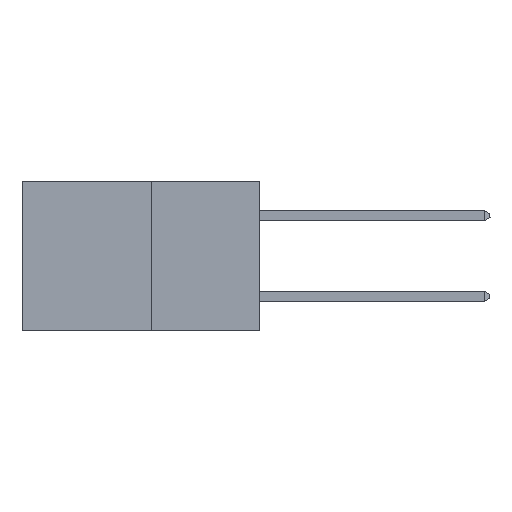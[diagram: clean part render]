
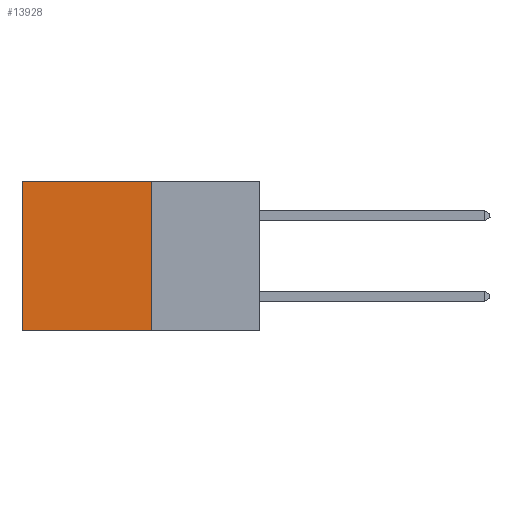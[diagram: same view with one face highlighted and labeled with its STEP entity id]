
A CAD part, left-side view. The second image highlights one B-rep face of the part: STEP entity #13928.
In plain terms, the highlighted planar face has unit normal (-1, 0, 0).
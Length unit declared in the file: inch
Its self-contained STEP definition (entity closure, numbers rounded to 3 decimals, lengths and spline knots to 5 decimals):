
#190 = EDGE_CURVE ( 'NONE', #4713, #26389, #25312, .T. ) ;
#2815 = VECTOR ( 'NONE', #17369, 39.37008 ) ;
#3020 = DIRECTION ( 'NONE',  ( 0., 0., -1. ) ) ;
#3487 = LINE ( 'NONE', #23505, #2815 ) ;
#4713 = VERTEX_POINT ( 'NONE', #15309 ) ;
#4972 = LINE ( 'NONE', #18026, #16426 ) ;
#5358 = CARTESIAN_POINT ( 'NONE',  ( 0.277, 0.27, 0. ) ) ;
#5372 = AXIS2_PLACEMENT_3D ( 'NONE', #22694, #10097, #24792 ) ;
#5730 = PLANE ( 'NONE',  #5372 ) ;
#5751 = LINE ( 'NONE', #5358, #17170 ) ;
#6756 = EDGE_CURVE ( 'NONE', #11425, #4713, #3487, .T. ) ;
#9179 = FACE_OUTER_BOUND ( 'NONE', #25872, .T. ) ;
#9618 = CARTESIAN_POINT ( 'NONE',  ( 0.277, 0.59, -0.37 ) ) ;
#9659 = DIRECTION ( 'NONE',  ( 0., 1., 0. ) ) ;
#10097 = DIRECTION ( 'NONE',  ( 1., 0., 0. ) ) ;
#11425 = VERTEX_POINT ( 'NONE', #22113 ) ;
#12475 = CARTESIAN_POINT ( 'NONE',  ( 0.277, 0.59, 0. ) ) ;
#13928 = ADVANCED_FACE ( 'NONE', ( #9179 ), #5730, .F. ) ;
#15016 = EDGE_CURVE ( 'NONE', #21531, #26389, #4972, .T. ) ;
#15309 = CARTESIAN_POINT ( 'NONE',  ( 0.277, 0.27, -0.37 ) ) ;
#15899 = DIRECTION ( 'NONE',  ( 0., 1., 0. ) ) ;
#16426 = VECTOR ( 'NONE', #3020, 39.37008 ) ;
#17170 = VECTOR ( 'NONE', #9659, 39.37008 ) ;
#17369 = DIRECTION ( 'NONE',  ( 0., 0., -1. ) ) ;
#17958 = ORIENTED_EDGE ( 'NONE', *, *, #190, .F. ) ;
#18026 = CARTESIAN_POINT ( 'NONE',  ( 0.277, 0.59, -0.37 ) ) ;
#18248 = ORIENTED_EDGE ( 'NONE', *, *, #6756, .F. ) ;
#19142 = VECTOR ( 'NONE', #15899, 39.37008 ) ;
#19360 = EDGE_CURVE ( 'NONE', #11425, #21531, #5751, .T. ) ;
#21357 = CARTESIAN_POINT ( 'NONE',  ( 0.277, 0.27, -0.37 ) ) ;
#21531 = VERTEX_POINT ( 'NONE', #12475 ) ;
#22113 = CARTESIAN_POINT ( 'NONE',  ( 0.277, 0.27, 0. ) ) ;
#22694 = CARTESIAN_POINT ( 'NONE',  ( 0.277, 0.27, -0.37 ) ) ;
#23505 = CARTESIAN_POINT ( 'NONE',  ( 0.277, 0.27, -0.37 ) ) ;
#23735 = ORIENTED_EDGE ( 'NONE', *, *, #19360, .T. ) ;
#24792 = DIRECTION ( 'NONE',  ( 0., 0., -1. ) ) ;
#25312 = LINE ( 'NONE', #21357, #19142 ) ;
#25872 = EDGE_LOOP ( 'NONE', ( #27030, #17958, #18248, #23735 ) ) ;
#26389 = VERTEX_POINT ( 'NONE', #9618 ) ;
#27030 = ORIENTED_EDGE ( 'NONE', *, *, #15016, .T. ) ;
